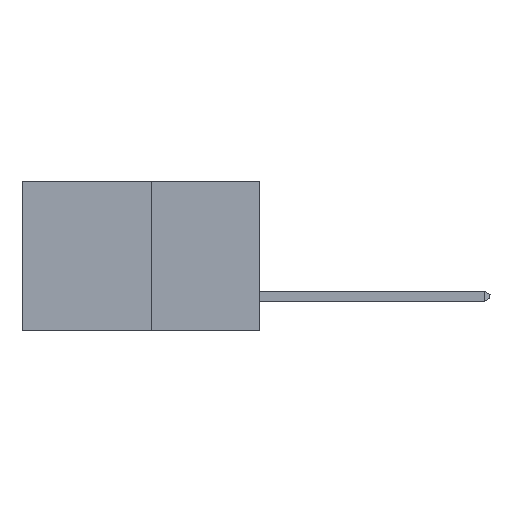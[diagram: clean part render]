
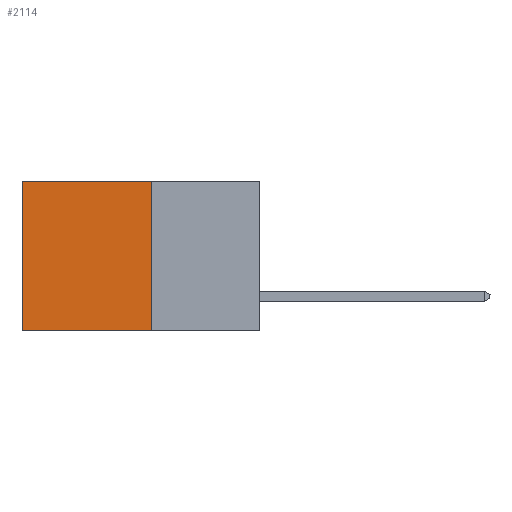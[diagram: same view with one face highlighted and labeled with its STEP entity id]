
A CAD part, left-side view. The second image highlights one B-rep face of the part: STEP entity #2114.
In plain terms, the highlighted planar face has unit normal (-1, 0, 0).
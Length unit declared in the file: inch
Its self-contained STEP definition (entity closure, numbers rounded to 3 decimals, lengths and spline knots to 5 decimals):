
#118 = EDGE_LOOP ( 'NONE', ( #16402, #13168, #9765, #16239 ) ) ;
#932 = VECTOR ( 'NONE', #4363, 39.37008 ) ;
#971 = PLANE ( 'NONE',  #2735 ) ;
#999 = VERTEX_POINT ( 'NONE', #16100 ) ;
#1007 = DIRECTION ( 'NONE',  ( 0., 0., -1. ) ) ;
#2114 = ADVANCED_FACE ( 'NONE', ( #11403 ), #971, .F. ) ;
#2424 = CARTESIAN_POINT ( 'NONE',  ( 0.277, 0.59, -0.37 ) ) ;
#2735 = AXIS2_PLACEMENT_3D ( 'NONE', #5158, #8430, #1007 ) ;
#2833 = EDGE_CURVE ( 'NONE', #4939, #999, #14956, .T. ) ;
#2883 = CARTESIAN_POINT ( 'NONE',  ( 0.277, 0.27, -0.37 ) ) ;
#3137 = CARTESIAN_POINT ( 'NONE',  ( 0.277, 0.27, 0. ) ) ;
#4246 = DIRECTION ( 'NONE',  ( 0., 1., 0. ) ) ;
#4363 = DIRECTION ( 'NONE',  ( 0., 0., -1. ) ) ;
#4406 = LINE ( 'NONE', #2883, #11215 ) ;
#4939 = VERTEX_POINT ( 'NONE', #6680 ) ;
#5158 = CARTESIAN_POINT ( 'NONE',  ( 0.277, 0.27, -0.37 ) ) ;
#5703 = CARTESIAN_POINT ( 'NONE',  ( 0.277, 0.27, -0.37 ) ) ;
#6211 = VERTEX_POINT ( 'NONE', #3137 ) ;
#6680 = CARTESIAN_POINT ( 'NONE',  ( 0.277, 0.59, 0. ) ) ;
#8237 = LINE ( 'NONE', #5703, #932 ) ;
#8430 = DIRECTION ( 'NONE',  ( 1., 0., 0. ) ) ;
#8480 = LINE ( 'NONE', #13113, #15066 ) ;
#9765 = ORIENTED_EDGE ( 'NONE', *, *, #10978, .F. ) ;
#9851 = DIRECTION ( 'NONE',  ( 0., 0., -1. ) ) ;
#9954 = EDGE_CURVE ( 'NONE', #15963, #999, #4406, .T. ) ;
#10363 = EDGE_CURVE ( 'NONE', #6211, #4939, #8480, .T. ) ;
#10978 = EDGE_CURVE ( 'NONE', #6211, #15963, #8237, .T. ) ;
#11215 = VECTOR ( 'NONE', #4246, 39.37008 ) ;
#11403 = FACE_OUTER_BOUND ( 'NONE', #118, .T. ) ;
#13113 = CARTESIAN_POINT ( 'NONE',  ( 0.277, 0.27, 0. ) ) ;
#13168 = ORIENTED_EDGE ( 'NONE', *, *, #9954, .F. ) ;
#13853 = CARTESIAN_POINT ( 'NONE',  ( 0.277, 0.27, -0.37 ) ) ;
#14431 = DIRECTION ( 'NONE',  ( 0., 1., 0. ) ) ;
#14555 = VECTOR ( 'NONE', #9851, 39.37008 ) ;
#14956 = LINE ( 'NONE', #2424, #14555 ) ;
#15066 = VECTOR ( 'NONE', #14431, 39.37008 ) ;
#15963 = VERTEX_POINT ( 'NONE', #13853 ) ;
#16100 = CARTESIAN_POINT ( 'NONE',  ( 0.277, 0.59, -0.37 ) ) ;
#16239 = ORIENTED_EDGE ( 'NONE', *, *, #10363, .T. ) ;
#16402 = ORIENTED_EDGE ( 'NONE', *, *, #2833, .T. ) ;
